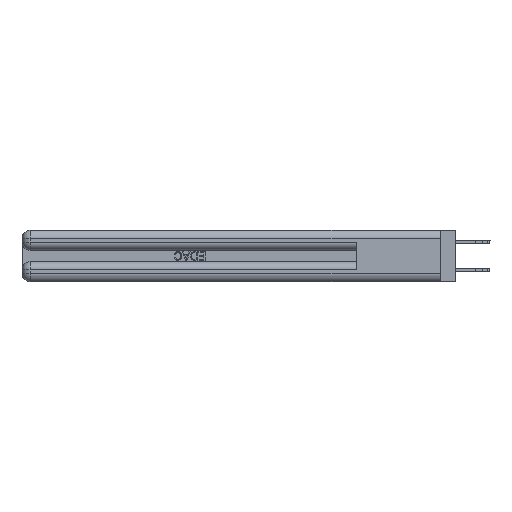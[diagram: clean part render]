
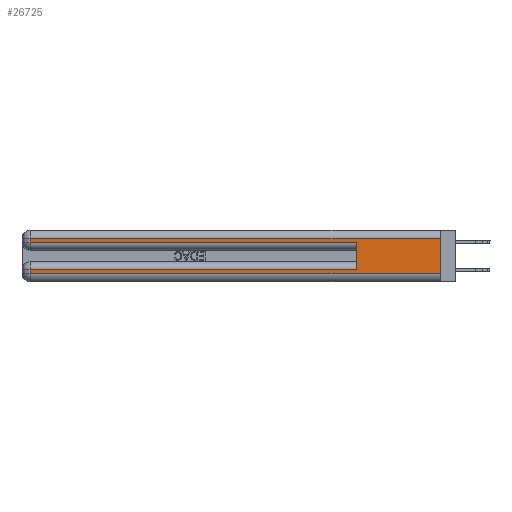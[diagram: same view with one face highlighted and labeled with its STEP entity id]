
A CAD part, left-side view. The second image highlights one B-rep face of the part: STEP entity #26725.
In plain terms, the highlighted planar face has unit normal (-1, 0, 0).
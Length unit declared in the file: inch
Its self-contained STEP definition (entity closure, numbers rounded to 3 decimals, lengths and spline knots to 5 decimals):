
#118 = ORIENTED_EDGE ( 'NONE', *, *, #10210, .F. ) ;
#226 = DIRECTION ( 'NONE',  ( 0., -1., 0. ) ) ;
#305 = LINE ( 'NONE', #5112, #37500 ) ;
#625 = DIRECTION ( 'NONE',  ( 0., 0., 1. ) ) ;
#725 = DIRECTION ( 'NONE',  ( 0., 0., -1. ) ) ;
#888 = ORIENTED_EDGE ( 'NONE', *, *, #19515, .T. ) ;
#913 = ORIENTED_EDGE ( 'NONE', *, *, #2841, .T. ) ;
#1082 = CARTESIAN_POINT ( 'NONE',  ( 0., 0., 0.06 ) ) ;
#1176 = VERTEX_POINT ( 'NONE', #4954 ) ;
#1753 = VECTOR ( 'NONE', #226, 39.37008 ) ;
#2021 = VERTEX_POINT ( 'NONE', #23138 ) ;
#2471 = EDGE_CURVE ( 'NONE', #36122, #22106, #38456, .T. ) ;
#2841 = EDGE_CURVE ( 'NONE', #1176, #2021, #37427, .T. ) ;
#2935 = CARTESIAN_POINT ( 'NONE',  ( 0., 0.6, 0.085 ) ) ;
#3524 = CARTESIAN_POINT ( 'NONE',  ( 0., 0., 0.31 ) ) ;
#3947 = CARTESIAN_POINT ( 'NONE',  ( 0., 2.94, 0.37 ) ) ;
#4360 = EDGE_CURVE ( 'NONE', #36122, #5331, #26400, .T. ) ;
#4954 = CARTESIAN_POINT ( 'NONE',  ( 0., 2.94, 0.085 ) ) ;
#5112 = CARTESIAN_POINT ( 'NONE',  ( 0., 0., 0.285 ) ) ;
#5270 = VECTOR ( 'NONE', #13335, 39.37008 ) ;
#5331 = VERTEX_POINT ( 'NONE', #1082 ) ;
#5892 = VECTOR ( 'NONE', #23862, 39.37008 ) ;
#6814 = EDGE_CURVE ( 'NONE', #13898, #1176, #37312, .T. ) ;
#7034 = ORIENTED_EDGE ( 'NONE', *, *, #4360, .F. ) ;
#8507 = DIRECTION ( 'NONE',  ( 0., -1., 0. ) ) ;
#8824 = LINE ( 'NONE', #39055, #1753 ) ;
#9231 = PLANE ( 'NONE',  #27098 ) ;
#9466 = CARTESIAN_POINT ( 'NONE',  ( 0., 0., 0.37 ) ) ;
#10210 = EDGE_CURVE ( 'NONE', #13898, #33291, #39956, .T. ) ;
#11454 = VECTOR ( 'NONE', #725, 39.37008 ) ;
#11570 = EDGE_CURVE ( 'NONE', #22106, #27108, #12801, .T. ) ;
#11580 = ORIENTED_EDGE ( 'NONE', *, *, #11570, .T. ) ;
#12801 = LINE ( 'NONE', #3947, #15865 ) ;
#13058 = DIRECTION ( 'NONE',  ( 1., 0., 0. ) ) ;
#13335 = DIRECTION ( 'NONE',  ( 0., 1., 0. ) ) ;
#13898 = VERTEX_POINT ( 'NONE', #2935 ) ;
#14728 = CARTESIAN_POINT ( 'NONE',  ( 0., 0., 0.31 ) ) ;
#15725 = DIRECTION ( 'NONE',  ( 0., 0., -1. ) ) ;
#15865 = VECTOR ( 'NONE', #30391, 39.37008 ) ;
#16545 = CARTESIAN_POINT ( 'NONE',  ( 0., 0.6, 0.145 ) ) ;
#17669 = EDGE_CURVE ( 'NONE', #27108, #33291, #305, .T. ) ;
#19470 = CARTESIAN_POINT ( 'NONE',  ( 0., 0., 0.37 ) ) ;
#19515 = EDGE_CURVE ( 'NONE', #2021, #5331, #8824, .T. ) ;
#22106 = VERTEX_POINT ( 'NONE', #28901 ) ;
#23138 = CARTESIAN_POINT ( 'NONE',  ( 0., 2.94, 0.06 ) ) ;
#23862 = DIRECTION ( 'NONE',  ( 0., 1., 0. ) ) ;
#26400 = LINE ( 'NONE', #9466, #35498 ) ;
#26456 = EDGE_LOOP ( 'NONE', ( #7034, #34914, #11580, #27503, #118, #31155, #913, #888 ) ) ;
#26725 = ADVANCED_FACE ( 'NONE', ( #37601 ), #9231, .F. ) ;
#27098 = AXIS2_PLACEMENT_3D ( 'NONE', #19470, #13058, #38677 ) ;
#27108 = VERTEX_POINT ( 'NONE', #31517 ) ;
#27503 = ORIENTED_EDGE ( 'NONE', *, *, #17669, .T. ) ;
#28901 = CARTESIAN_POINT ( 'NONE',  ( 0., 2.94, 0.31 ) ) ;
#29576 = CARTESIAN_POINT ( 'NONE',  ( 0., 0., 0.085 ) ) ;
#30391 = DIRECTION ( 'NONE',  ( 0., 0., -1. ) ) ;
#31155 = ORIENTED_EDGE ( 'NONE', *, *, #6814, .T. ) ;
#31517 = CARTESIAN_POINT ( 'NONE',  ( 0., 2.94, 0.285 ) ) ;
#32203 = CARTESIAN_POINT ( 'NONE',  ( 0., 0.6, 0.285 ) ) ;
#33291 = VERTEX_POINT ( 'NONE', #32203 ) ;
#34914 = ORIENTED_EDGE ( 'NONE', *, *, #2471, .T. ) ;
#35366 = VECTOR ( 'NONE', #625, 39.37008 ) ;
#35498 = VECTOR ( 'NONE', #15725, 39.37008 ) ;
#36122 = VERTEX_POINT ( 'NONE', #14728 ) ;
#37312 = LINE ( 'NONE', #29576, #5270 ) ;
#37427 = LINE ( 'NONE', #40106, #11454 ) ;
#37500 = VECTOR ( 'NONE', #8507, 39.37008 ) ;
#37601 = FACE_OUTER_BOUND ( 'NONE', #26456, .T. ) ;
#38456 = LINE ( 'NONE', #3524, #5892 ) ;
#38677 = DIRECTION ( 'NONE',  ( 0., 0., -1. ) ) ;
#39055 = CARTESIAN_POINT ( 'NONE',  ( 0., 0., 0.06 ) ) ;
#39956 = LINE ( 'NONE', #16545, #35366 ) ;
#40106 = CARTESIAN_POINT ( 'NONE',  ( 0., 2.94, 0.37 ) ) ;
